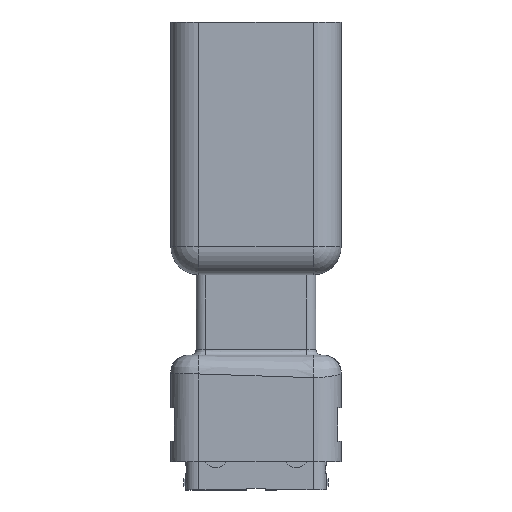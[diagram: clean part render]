
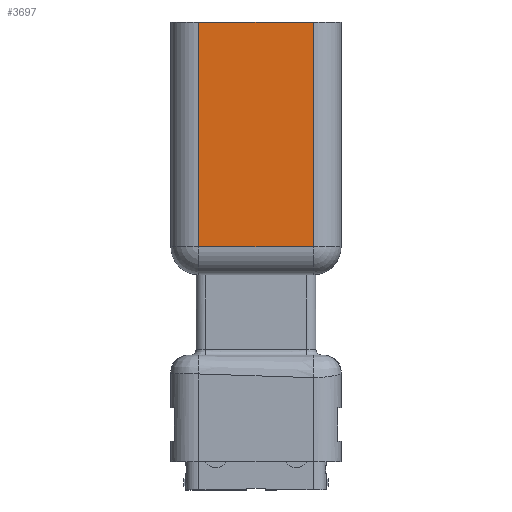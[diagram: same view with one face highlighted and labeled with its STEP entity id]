
A CAD part, front view. The second image highlights one B-rep face of the part: STEP entity #3697.
In plain terms, the highlighted planar face has unit normal (0, -1, 0).
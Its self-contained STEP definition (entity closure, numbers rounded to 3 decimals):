
#382 = EDGE_LOOP ( 'NONE', ( #13762, #2963, #4823, #12442 ) ) ;
#763 = DIRECTION ( 'NONE',  ( 0., 0., -1. ) ) ;
#852 = DIRECTION ( 'NONE',  ( 1., 0., 0. ) ) ;
#948 = CARTESIAN_POINT ( 'NONE',  ( -3.05, -3.955, 13.5 ) ) ;
#977 = CARTESIAN_POINT ( 'NONE',  ( 3.05, -3.955, 13.5 ) ) ;
#2424 = VERTEX_POINT ( 'NONE', #4514 ) ;
#2963 = ORIENTED_EDGE ( 'NONE', *, *, #5727, .T. ) ;
#3697 = ADVANCED_FACE ( 'NONE', ( #17675 ), #6293, .F. ) ;
#4315 = CARTESIAN_POINT ( 'NONE',  ( -3.05, -3.955, 1.5 ) ) ;
#4483 = VERTEX_POINT ( 'NONE', #4315 ) ;
#4514 = CARTESIAN_POINT ( 'NONE',  ( -3.05, -3.955, 13.5 ) ) ;
#4823 = ORIENTED_EDGE ( 'NONE', *, *, #7619, .F. ) ;
#5378 = DIRECTION ( 'NONE',  ( 0., 1., 0. ) ) ;
#5727 = EDGE_CURVE ( 'NONE', #4483, #13223, #7933, .T. ) ;
#6293 = PLANE ( 'NONE',  #7787 ) ;
#6930 = EDGE_CURVE ( 'NONE', #2424, #15105, #14398, .T. ) ;
#7619 = EDGE_CURVE ( 'NONE', #15105, #13223, #12767, .T. ) ;
#7787 = AXIS2_PLACEMENT_3D ( 'NONE', #12008, #5378, #16160 ) ;
#7933 = LINE ( 'NONE', #12220, #12763 ) ;
#8382 = DIRECTION ( 'NONE',  ( 0., 0., -1. ) ) ;
#8446 = CARTESIAN_POINT ( 'NONE',  ( 3.05, -3.955, 1.5 ) ) ;
#10349 = LINE ( 'NONE', #14735, #10513 ) ;
#10513 = VECTOR ( 'NONE', #763, 1000. ) ;
#12008 = CARTESIAN_POINT ( 'NONE',  ( -3.05, -3.955, 13.5 ) ) ;
#12220 = CARTESIAN_POINT ( 'NONE',  ( -3.05, -3.955, 1.5 ) ) ;
#12442 = ORIENTED_EDGE ( 'NONE', *, *, #6930, .F. ) ;
#12763 = VECTOR ( 'NONE', #15090, 1000. ) ;
#12767 = LINE ( 'NONE', #15368, #14894 ) ;
#13223 = VERTEX_POINT ( 'NONE', #8446 ) ;
#13762 = ORIENTED_EDGE ( 'NONE', *, *, #17044, .T. ) ;
#14377 = VECTOR ( 'NONE', #852, 1000. ) ;
#14398 = LINE ( 'NONE', #948, #14377 ) ;
#14735 = CARTESIAN_POINT ( 'NONE',  ( -3.05, -3.955, 13.5 ) ) ;
#14894 = VECTOR ( 'NONE', #8382, 1000. ) ;
#15090 = DIRECTION ( 'NONE',  ( 1., 0., 0. ) ) ;
#15105 = VERTEX_POINT ( 'NONE', #977 ) ;
#15368 = CARTESIAN_POINT ( 'NONE',  ( 3.05, -3.955, 13.5 ) ) ;
#16160 = DIRECTION ( 'NONE',  ( 0., 0., 1. ) ) ;
#17044 = EDGE_CURVE ( 'NONE', #2424, #4483, #10349, .T. ) ;
#17675 = FACE_OUTER_BOUND ( 'NONE', #382, .T. ) ;
